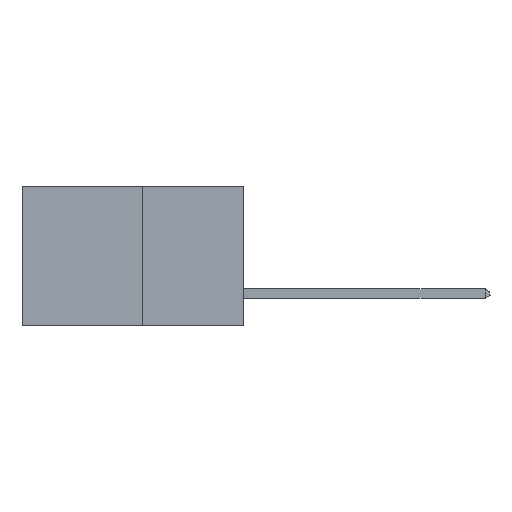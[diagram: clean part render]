
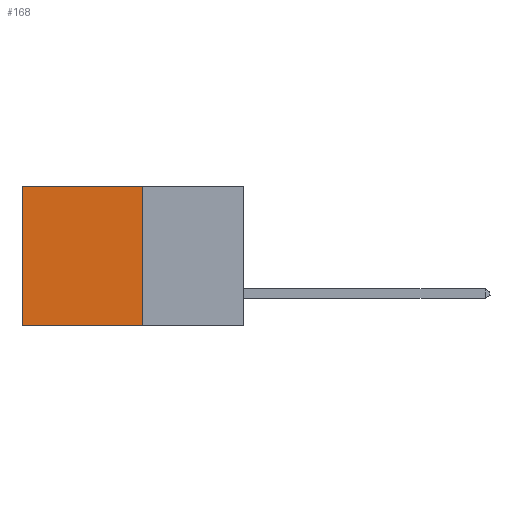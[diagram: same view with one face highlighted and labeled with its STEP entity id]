
A CAD part, left-side view. The second image highlights one B-rep face of the part: STEP entity #168.
In plain terms, the highlighted planar face has unit normal (-1, 0, 0).
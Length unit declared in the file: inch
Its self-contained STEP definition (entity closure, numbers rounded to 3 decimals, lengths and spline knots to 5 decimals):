
#13 = VERTEX_POINT ( 'NONE', #5616 ) ;
#110 = DIRECTION ( 'NONE',  ( 0., 0., -1. ) ) ;
#168 = ADVANCED_FACE ( 'NONE', ( #546 ), #5238, .F. ) ;
#546 = FACE_OUTER_BOUND ( 'NONE', #1938, .T. ) ;
#1182 = VECTOR ( 'NONE', #3586, 39.37008 ) ;
#1938 = EDGE_LOOP ( 'NONE', ( #9771, #3521, #9268, #8669 ) ) ;
#2051 = VERTEX_POINT ( 'NONE', #4006 ) ;
#2168 = LINE ( 'NONE', #3571, #11469 ) ;
#3182 = VECTOR ( 'NONE', #10715, 39.37008 ) ;
#3521 = ORIENTED_EDGE ( 'NONE', *, *, #4403, .F. ) ;
#3571 = CARTESIAN_POINT ( 'NONE',  ( 0.277, 0.27, -0.37 ) ) ;
#3586 = DIRECTION ( 'NONE',  ( 0., 1., 0. ) ) ;
#4006 = CARTESIAN_POINT ( 'NONE',  ( 0.277, 0.59, -0.37 ) ) ;
#4403 = EDGE_CURVE ( 'NONE', #6070, #2051, #8137, .T. ) ;
#5238 = PLANE ( 'NONE',  #10617 ) ;
#5616 = CARTESIAN_POINT ( 'NONE',  ( 0.277, 0.27, 0. ) ) ;
#5694 = VERTEX_POINT ( 'NONE', #8132 ) ;
#6070 = VERTEX_POINT ( 'NONE', #10670 ) ;
#6522 = CARTESIAN_POINT ( 'NONE',  ( 0.277, 0.27, 0. ) ) ;
#7339 = VECTOR ( 'NONE', #110, 39.37008 ) ;
#8132 = CARTESIAN_POINT ( 'NONE',  ( 0.277, 0.59, 0. ) ) ;
#8137 = LINE ( 'NONE', #8339, #1182 ) ;
#8304 = CARTESIAN_POINT ( 'NONE',  ( 0.277, 0.59, -0.37 ) ) ;
#8339 = CARTESIAN_POINT ( 'NONE',  ( 0.277, 0.27, -0.37 ) ) ;
#8402 = CARTESIAN_POINT ( 'NONE',  ( 0.277, 0.27, -0.37 ) ) ;
#8451 = DIRECTION ( 'NONE',  ( 1., 0., 0. ) ) ;
#8669 = ORIENTED_EDGE ( 'NONE', *, *, #11064, .T. ) ;
#9247 = EDGE_CURVE ( 'NONE', #5694, #2051, #11475, .T. ) ;
#9268 = ORIENTED_EDGE ( 'NONE', *, *, #10275, .F. ) ;
#9365 = DIRECTION ( 'NONE',  ( 0., 0., -1. ) ) ;
#9771 = ORIENTED_EDGE ( 'NONE', *, *, #9247, .T. ) ;
#10117 = LINE ( 'NONE', #6522, #3182 ) ;
#10275 = EDGE_CURVE ( 'NONE', #13, #6070, #2168, .T. ) ;
#10617 = AXIS2_PLACEMENT_3D ( 'NONE', #8402, #8451, #9365 ) ;
#10670 = CARTESIAN_POINT ( 'NONE',  ( 0.277, 0.27, -0.37 ) ) ;
#10715 = DIRECTION ( 'NONE',  ( 0., 1., 0. ) ) ;
#11064 = EDGE_CURVE ( 'NONE', #13, #5694, #10117, .T. ) ;
#11344 = DIRECTION ( 'NONE',  ( 0., 0., -1. ) ) ;
#11469 = VECTOR ( 'NONE', #11344, 39.37008 ) ;
#11475 = LINE ( 'NONE', #8304, #7339 ) ;
